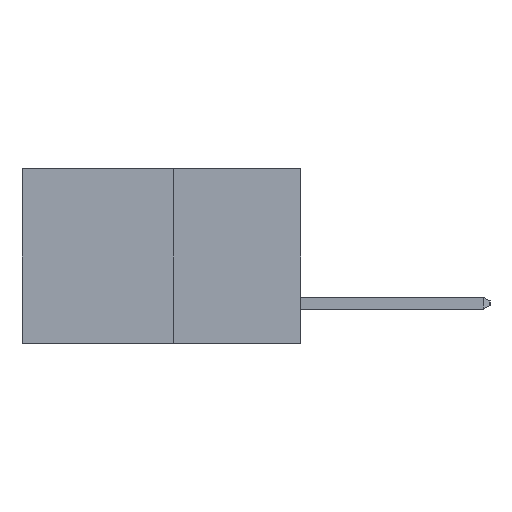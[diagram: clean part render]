
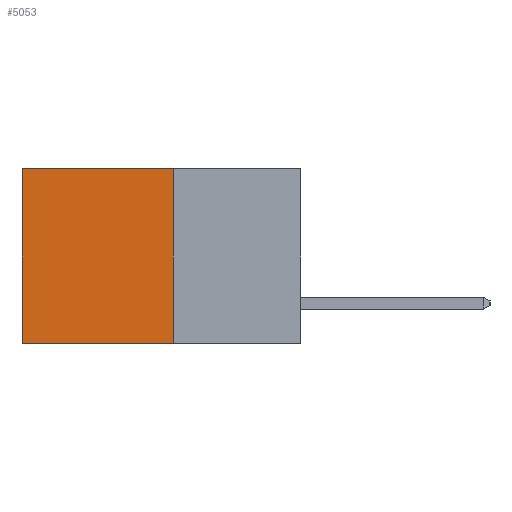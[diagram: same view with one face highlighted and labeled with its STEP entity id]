
A CAD part, left-side view. The second image highlights one B-rep face of the part: STEP entity #5053.
In plain terms, the highlighted planar face has unit normal (-1, 0, 0).
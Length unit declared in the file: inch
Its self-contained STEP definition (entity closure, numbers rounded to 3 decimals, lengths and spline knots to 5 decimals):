
#206 = PLANE ( 'NONE',  #4659 ) ;
#366 = VECTOR ( 'NONE', #10576, 39.37008 ) ;
#955 = EDGE_CURVE ( 'NONE', #8421, #13027, #3600, .T. ) ;
#1689 = ORIENTED_EDGE ( 'NONE', *, *, #11211, .F. ) ;
#2910 = CARTESIAN_POINT ( 'NONE',  ( 0.277, 0.27, -0.37 ) ) ;
#3143 = VERTEX_POINT ( 'NONE', #2910 ) ;
#3201 = DIRECTION ( 'NONE',  ( 0., 0., -1. ) ) ;
#3501 = LINE ( 'NONE', #10587, #366 ) ;
#3600 = LINE ( 'NONE', #10430, #9235 ) ;
#3712 = ORIENTED_EDGE ( 'NONE', *, *, #8284, .T. ) ;
#3965 = EDGE_LOOP ( 'NONE', ( #3712, #1689, #8086, #11088 ) ) ;
#4238 = VECTOR ( 'NONE', #10343, 39.37008 ) ;
#4659 = AXIS2_PLACEMENT_3D ( 'NONE', #7116, #9226, #8165 ) ;
#4686 = CARTESIAN_POINT ( 'NONE',  ( 0.277, 0.27, -0.37 ) ) ;
#5053 = ADVANCED_FACE ( 'NONE', ( #10978 ), #206, .F. ) ;
#5895 = EDGE_CURVE ( 'NONE', #8421, #3143, #10951, .T. ) ;
#6977 = CARTESIAN_POINT ( 'NONE',  ( 0.277, 0.59, -0.37 ) ) ;
#7116 = CARTESIAN_POINT ( 'NONE',  ( 0.277, 0.27, -0.37 ) ) ;
#7776 = VERTEX_POINT ( 'NONE', #6977 ) ;
#8086 = ORIENTED_EDGE ( 'NONE', *, *, #5895, .F. ) ;
#8165 = DIRECTION ( 'NONE',  ( 0., 0., -1. ) ) ;
#8284 = EDGE_CURVE ( 'NONE', #13027, #7776, #13126, .T. ) ;
#8421 = VERTEX_POINT ( 'NONE', #9069 ) ;
#9069 = CARTESIAN_POINT ( 'NONE',  ( 0.277, 0.27, 0. ) ) ;
#9226 = DIRECTION ( 'NONE',  ( 1., 0., 0. ) ) ;
#9235 = VECTOR ( 'NONE', #10445, 39.37008 ) ;
#10343 = DIRECTION ( 'NONE',  ( 0., 0., -1. ) ) ;
#10430 = CARTESIAN_POINT ( 'NONE',  ( 0.277, 0.27, 0. ) ) ;
#10445 = DIRECTION ( 'NONE',  ( 0., 1., 0. ) ) ;
#10575 = CARTESIAN_POINT ( 'NONE',  ( 0.277, 0.59, -0.37 ) ) ;
#10576 = DIRECTION ( 'NONE',  ( 0., 1., 0. ) ) ;
#10587 = CARTESIAN_POINT ( 'NONE',  ( 0.277, 0.27, -0.37 ) ) ;
#10613 = VECTOR ( 'NONE', #3201, 39.37008 ) ;
#10951 = LINE ( 'NONE', #4686, #10613 ) ;
#10978 = FACE_OUTER_BOUND ( 'NONE', #3965, .T. ) ;
#11088 = ORIENTED_EDGE ( 'NONE', *, *, #955, .T. ) ;
#11211 = EDGE_CURVE ( 'NONE', #3143, #7776, #3501, .T. ) ;
#11219 = CARTESIAN_POINT ( 'NONE',  ( 0.277, 0.59, 0. ) ) ;
#13027 = VERTEX_POINT ( 'NONE', #11219 ) ;
#13126 = LINE ( 'NONE', #10575, #4238 ) ;
